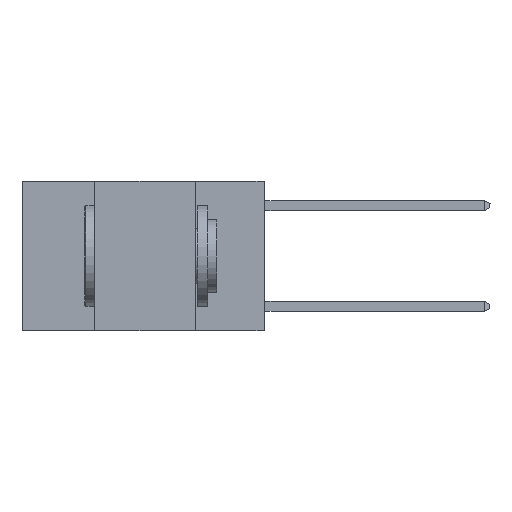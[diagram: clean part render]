
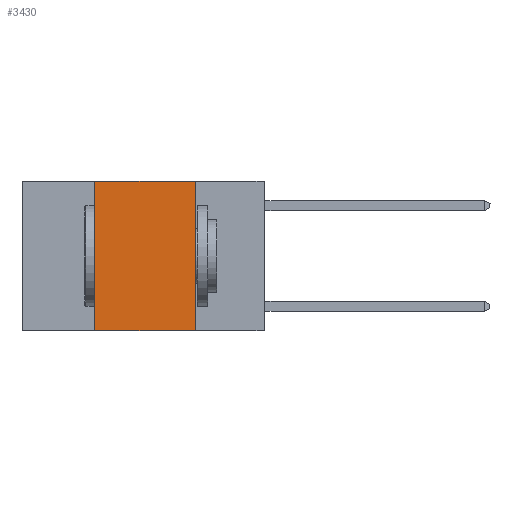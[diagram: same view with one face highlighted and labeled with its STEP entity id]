
A CAD part, left-side view. The second image highlights one B-rep face of the part: STEP entity #3430.
In plain terms, the highlighted planar face has unit normal (-1, 0, 0).
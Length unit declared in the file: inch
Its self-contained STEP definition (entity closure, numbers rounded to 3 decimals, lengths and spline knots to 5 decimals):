
#414 = CARTESIAN_POINT ( 'NONE',  ( 0., 0.42, -0.37 ) ) ;
#1677 = EDGE_CURVE ( 'NONE', #18208, #7878, #6677, .T. ) ;
#3017 = DIRECTION ( 'NONE',  ( 0., -1., 0. ) ) ;
#3430 = ADVANCED_FACE ( 'NONE', ( #16791 ), #9499, .F. ) ;
#4626 = DIRECTION ( 'NONE',  ( 0., 0., -1. ) ) ;
#6129 = CARTESIAN_POINT ( 'NONE',  ( 0., 0.6, 0. ) ) ;
#6317 = VECTOR ( 'NONE', #12989, 39.37008 ) ;
#6483 = EDGE_CURVE ( 'NONE', #18208, #17941, #8123, .T. ) ;
#6578 = LINE ( 'NONE', #15100, #11728 ) ;
#6677 = LINE ( 'NONE', #8710, #8647 ) ;
#7124 = CARTESIAN_POINT ( 'NONE',  ( 0., 0.17, -0.37 ) ) ;
#7878 = VERTEX_POINT ( 'NONE', #7124 ) ;
#8123 = LINE ( 'NONE', #11982, #18042 ) ;
#8350 = DIRECTION ( 'NONE',  ( 0., 0., 1. ) ) ;
#8647 = VECTOR ( 'NONE', #11655, 39.37008 ) ;
#8710 = CARTESIAN_POINT ( 'NONE',  ( 0., 0.6, -0.37 ) ) ;
#8853 = VERTEX_POINT ( 'NONE', #19911 ) ;
#9499 = PLANE ( 'NONE',  #13577 ) ;
#10672 = EDGE_CURVE ( 'NONE', #17941, #8853, #6578, .T. ) ;
#11655 = DIRECTION ( 'NONE',  ( 0., -1., 0. ) ) ;
#11728 = VECTOR ( 'NONE', #3017, 39.37008 ) ;
#11982 = CARTESIAN_POINT ( 'NONE',  ( 0., 0.42, 0. ) ) ;
#12385 = EDGE_LOOP ( 'NONE', ( #17946, #12606, #21117, #14846 ) ) ;
#12606 = ORIENTED_EDGE ( 'NONE', *, *, #10672, .F. ) ;
#12989 = DIRECTION ( 'NONE',  ( 0., 0., -1. ) ) ;
#13577 = AXIS2_PLACEMENT_3D ( 'NONE', #6129, #20199, #4626 ) ;
#14846 = ORIENTED_EDGE ( 'NONE', *, *, #1677, .T. ) ;
#15100 = CARTESIAN_POINT ( 'NONE',  ( 0., 0.6, 0. ) ) ;
#16791 = FACE_OUTER_BOUND ( 'NONE', #12385, .T. ) ;
#17941 = VERTEX_POINT ( 'NONE', #18298 ) ;
#17946 = ORIENTED_EDGE ( 'NONE', *, *, #18695, .F. ) ;
#18005 = LINE ( 'NONE', #21520, #6317 ) ;
#18042 = VECTOR ( 'NONE', #8350, 39.37008 ) ;
#18208 = VERTEX_POINT ( 'NONE', #414 ) ;
#18298 = CARTESIAN_POINT ( 'NONE',  ( 0., 0.42, 0. ) ) ;
#18695 = EDGE_CURVE ( 'NONE', #8853, #7878, #18005, .T. ) ;
#19911 = CARTESIAN_POINT ( 'NONE',  ( 0., 0.17, 0. ) ) ;
#20199 = DIRECTION ( 'NONE',  ( 1., 0., 0. ) ) ;
#21117 = ORIENTED_EDGE ( 'NONE', *, *, #6483, .F. ) ;
#21520 = CARTESIAN_POINT ( 'NONE',  ( 0., 0.17, 0. ) ) ;
